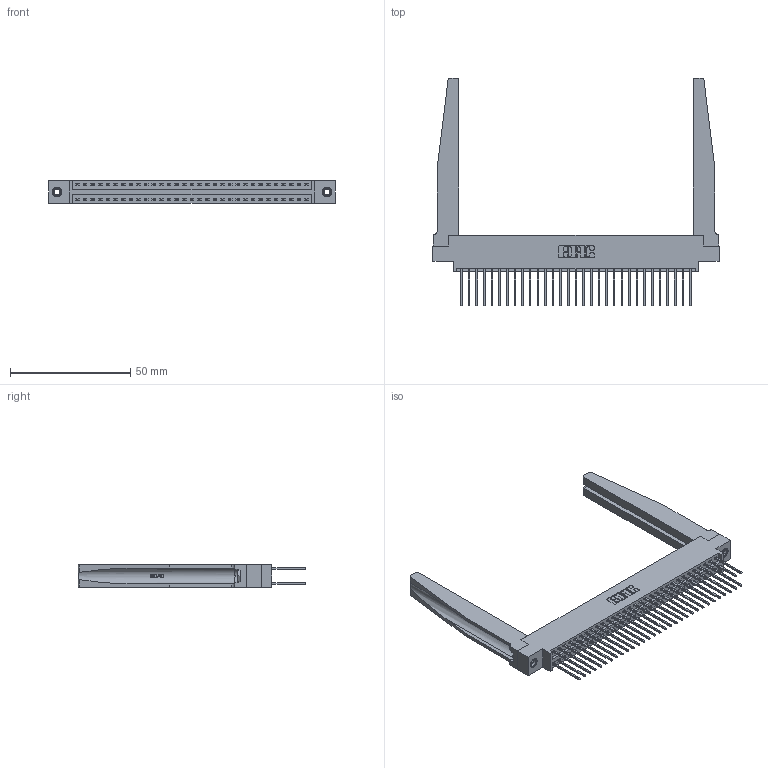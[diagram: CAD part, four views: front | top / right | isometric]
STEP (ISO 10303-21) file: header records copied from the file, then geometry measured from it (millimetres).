
FILE_DESCRIPTION (( 'STEP AP203' ), '1' );
FILE_NAME ('346-062-540-878.STEP', '2022-05-24T13:51:46', ( '' ), ( '' ), 'SwSTEP 2.0', 'SolidWorks 2020', '' );
FILE_SCHEMA (( 'CONFIG_CONTROL_DESIGN' ));
Length unit declared in the file: inch
Products named in the file (5): 346 Part_0.170 Offset - 0.156 Dia-TH; 345-292-001_345-293-140; 346-220-078_345-220-078; 345-250-001_345-250-001-102; 346-062-540-878
Assembly tree (67 placements, depth 2):
  346-062-540-878
    346 Part_0.170 Offset - 0.156 Dia-TH
    345-292-001_345-293-140  x62
    346-220-078_345-220-078  x2
    345-250-001_345-250-001-102  x2
Bounding box: 119 x 94.74 x 9.4 mm (x, y, z)
Volume: 18489.6 mm3; surface area: 23609.1 mm2
Topology: 67 solids, 67 shells, 3598 faces, 10595 edges, 6970 vertices
Faces by surface type: plane 2406, cylinder 1140, bspline 36, cone 12, torus 4
Entity records: 27026 total; most frequent: CARTESIAN_POINT 5413, ORIENTED_EDGE 4234, DIRECTION 3807, EDGE_CURVE 2117, VECTOR 1767, LINE 1767, VERTEX_POINT 1404, AXIS2_PLACEMENT_3D 1020
